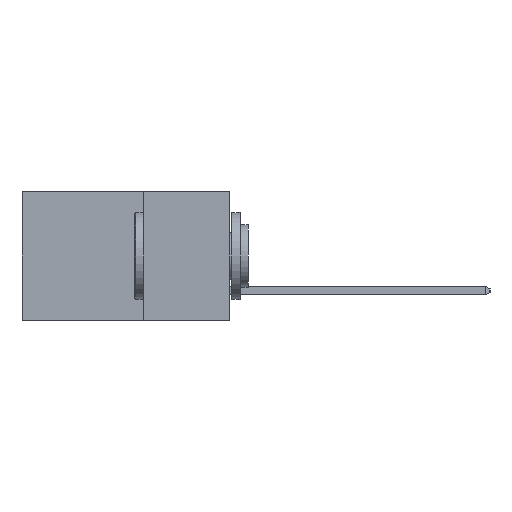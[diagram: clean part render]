
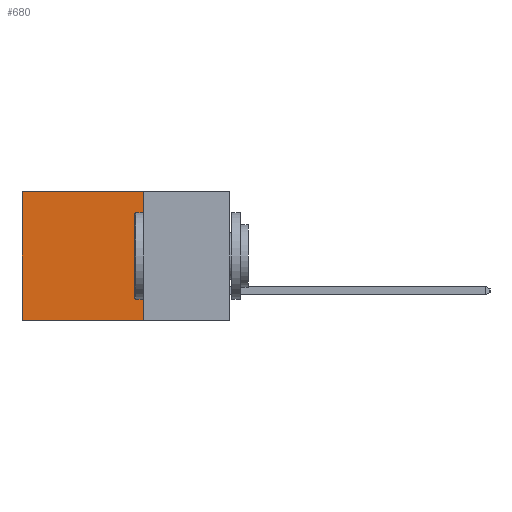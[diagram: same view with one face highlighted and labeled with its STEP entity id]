
A CAD part, left-side view. The second image highlights one B-rep face of the part: STEP entity #680.
In plain terms, the highlighted planar face has unit normal (-1, 0, 0).
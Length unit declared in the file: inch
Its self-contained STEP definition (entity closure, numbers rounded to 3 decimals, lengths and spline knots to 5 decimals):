
#6 = DIRECTION ( 'NONE',  ( 1., 0., 0. ) ) ;
#9 = DIRECTION ( 'NONE',  ( 0., 0., -1. ) ) ;
#123 = VERTEX_POINT ( 'NONE', #9992 ) ;
#394 = FACE_OUTER_BOUND ( 'NONE', #6664, .T. ) ;
#508 = CARTESIAN_POINT ( 'NONE',  ( 0.298, 0.25, 0. ) ) ;
#569 = ORIENTED_EDGE ( 'NONE', *, *, #2179, .T. ) ;
#680 = ADVANCED_FACE ( 'NONE', ( #394 ), #12712, .F. ) ;
#2136 = CARTESIAN_POINT ( 'NONE',  ( 0.298, 0.25, -0.37 ) ) ;
#2179 = EDGE_CURVE ( 'NONE', #123, #10909, #12583, .T. ) ;
#2712 = DIRECTION ( 'NONE',  ( 0., 1., 0. ) ) ;
#4005 = CARTESIAN_POINT ( 'NONE',  ( 0.298, 0.6, -0.37 ) ) ;
#4433 = VECTOR ( 'NONE', #2712, 39.37008 ) ;
#4974 = LINE ( 'NONE', #5912, #12742 ) ;
#5059 = EDGE_CURVE ( 'NONE', #10909, #5185, #6483, .T. ) ;
#5185 = VERTEX_POINT ( 'NONE', #4005 ) ;
#5500 = CARTESIAN_POINT ( 'NONE',  ( 0.298, 0.6, 0. ) ) ;
#5713 = ORIENTED_EDGE ( 'NONE', *, *, #13404, .F. ) ;
#5912 = CARTESIAN_POINT ( 'NONE',  ( 0.298, 0.25, 0. ) ) ;
#6483 = LINE ( 'NONE', #12935, #11915 ) ;
#6664 = EDGE_LOOP ( 'NONE', ( #12910, #5713, #8346, #569 ) ) ;
#6779 = LINE ( 'NONE', #12795, #12184 ) ;
#6789 = DIRECTION ( 'NONE',  ( 0., 1., 0. ) ) ;
#7902 = DIRECTION ( 'NONE',  ( 0., 0., -1. ) ) ;
#8346 = ORIENTED_EDGE ( 'NONE', *, *, #9636, .F. ) ;
#8394 = CARTESIAN_POINT ( 'NONE',  ( 0.298, 0.25, 0. ) ) ;
#9321 = VERTEX_POINT ( 'NONE', #2136 ) ;
#9636 = EDGE_CURVE ( 'NONE', #123, #9321, #4974, .T. ) ;
#9992 = CARTESIAN_POINT ( 'NONE',  ( 0.298, 0.25, 0. ) ) ;
#10084 = DIRECTION ( 'NONE',  ( 0., 0., -1. ) ) ;
#10909 = VERTEX_POINT ( 'NONE', #5500 ) ;
#11915 = VECTOR ( 'NONE', #7902, 39.37008 ) ;
#12184 = VECTOR ( 'NONE', #6789, 39.37008 ) ;
#12324 = AXIS2_PLACEMENT_3D ( 'NONE', #8394, #6, #9 ) ;
#12583 = LINE ( 'NONE', #508, #4433 ) ;
#12712 = PLANE ( 'NONE',  #12324 ) ;
#12742 = VECTOR ( 'NONE', #10084, 39.37008 ) ;
#12795 = CARTESIAN_POINT ( 'NONE',  ( 0.298, 0.25, -0.37 ) ) ;
#12910 = ORIENTED_EDGE ( 'NONE', *, *, #5059, .T. ) ;
#12935 = CARTESIAN_POINT ( 'NONE',  ( 0.298, 0.6, 0. ) ) ;
#13404 = EDGE_CURVE ( 'NONE', #9321, #5185, #6779, .T. ) ;
